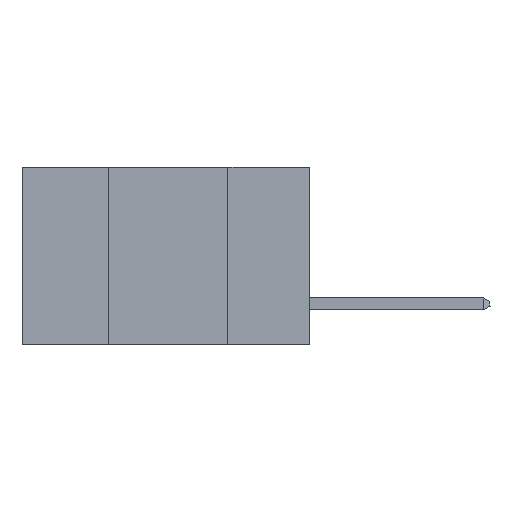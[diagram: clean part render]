
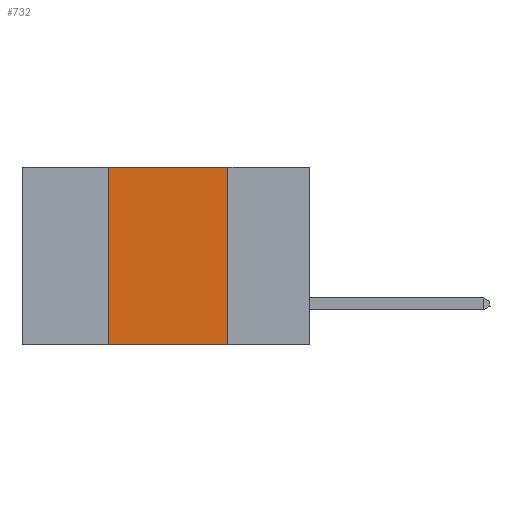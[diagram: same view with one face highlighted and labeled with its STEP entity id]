
A CAD part, left-side view. The second image highlights one B-rep face of the part: STEP entity #732.
In plain terms, the highlighted planar face has unit normal (-1, 0, 0).
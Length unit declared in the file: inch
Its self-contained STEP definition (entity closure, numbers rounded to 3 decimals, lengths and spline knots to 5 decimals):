
#732 = ADVANCED_FACE ( 'NONE', ( #44040 ), #13332, .F. ) ;
#1337 = EDGE_CURVE ( 'NONE', #16259, #4511, #31635, .T. ) ;
#2402 = CARTESIAN_POINT ( 'NONE',  ( 0., 0.42, 0. ) ) ;
#2529 = CARTESIAN_POINT ( 'NONE',  ( 0., 0.17, 0. ) ) ;
#4038 = DIRECTION ( 'NONE',  ( 0., -1., 0. ) ) ;
#4511 = VERTEX_POINT ( 'NONE', #41128 ) ;
#6724 = DIRECTION ( 'NONE',  ( 1., 0., 0. ) ) ;
#9496 = DIRECTION ( 'NONE',  ( 0., 0., -1. ) ) ;
#11252 = LINE ( 'NONE', #20502, #12338 ) ;
#11410 = ORIENTED_EDGE ( 'NONE', *, *, #1337, .F. ) ;
#11955 = CARTESIAN_POINT ( 'NONE',  ( 0., 0.42, -0.37 ) ) ;
#12338 = VECTOR ( 'NONE', #17288, 39.37008 ) ;
#13005 = VERTEX_POINT ( 'NONE', #11955 ) ;
#13332 = PLANE ( 'NONE',  #30661 ) ;
#13703 = CARTESIAN_POINT ( 'NONE',  ( 0., 0.17, 0. ) ) ;
#13809 = EDGE_CURVE ( 'NONE', #13005, #34078, #16970, .T. ) ;
#15697 = VECTOR ( 'NONE', #33832, 39.37008 ) ;
#16185 = LINE ( 'NONE', #18508, #31532 ) ;
#16259 = VERTEX_POINT ( 'NONE', #13703 ) ;
#16970 = LINE ( 'NONE', #17493, #28954 ) ;
#17288 = DIRECTION ( 'NONE',  ( 0., -1., 0. ) ) ;
#17493 = CARTESIAN_POINT ( 'NONE',  ( 0., 0.42, 0. ) ) ;
#18508 = CARTESIAN_POINT ( 'NONE',  ( 0., 0.6, -0.37 ) ) ;
#20502 = CARTESIAN_POINT ( 'NONE',  ( 0., 0.6, 0. ) ) ;
#27774 = CARTESIAN_POINT ( 'NONE',  ( 0., 0.6, 0. ) ) ;
#28954 = VECTOR ( 'NONE', #44803, 39.37008 ) ;
#29470 = ORIENTED_EDGE ( 'NONE', *, *, #44796, .F. ) ;
#30661 = AXIS2_PLACEMENT_3D ( 'NONE', #27774, #6724, #9496 ) ;
#31532 = VECTOR ( 'NONE', #4038, 39.37008 ) ;
#31635 = LINE ( 'NONE', #2529, #15697 ) ;
#33054 = ORIENTED_EDGE ( 'NONE', *, *, #13809, .F. ) ;
#33832 = DIRECTION ( 'NONE',  ( 0., 0., -1. ) ) ;
#34078 = VERTEX_POINT ( 'NONE', #2402 ) ;
#34435 = EDGE_LOOP ( 'NONE', ( #11410, #29470, #33054, #35522 ) ) ;
#35522 = ORIENTED_EDGE ( 'NONE', *, *, #37522, .T. ) ;
#37522 = EDGE_CURVE ( 'NONE', #13005, #4511, #16185, .T. ) ;
#41128 = CARTESIAN_POINT ( 'NONE',  ( 0., 0.17, -0.37 ) ) ;
#44040 = FACE_OUTER_BOUND ( 'NONE', #34435, .T. ) ;
#44796 = EDGE_CURVE ( 'NONE', #34078, #16259, #11252, .T. ) ;
#44803 = DIRECTION ( 'NONE',  ( 0., 0., 1. ) ) ;
